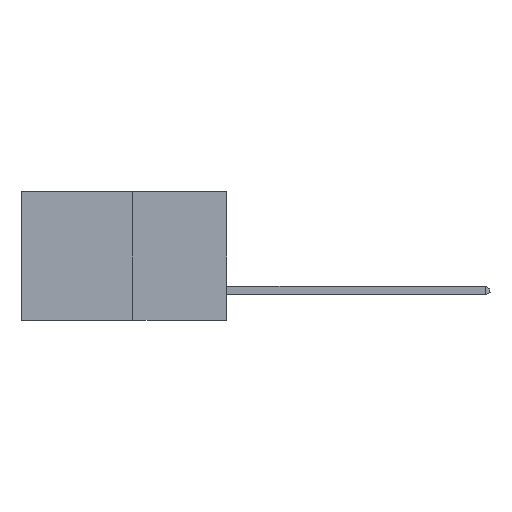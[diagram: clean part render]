
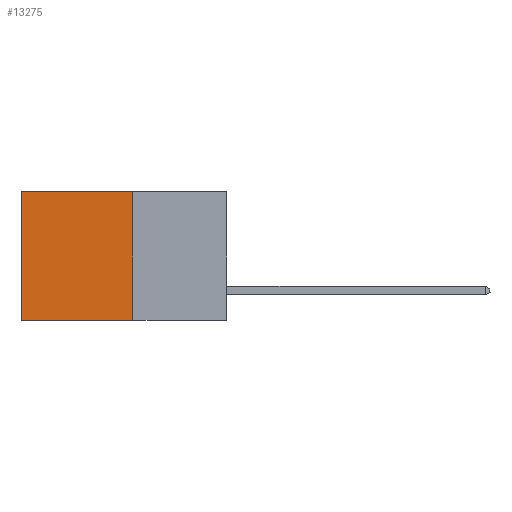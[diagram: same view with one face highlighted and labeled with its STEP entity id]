
A CAD part, left-side view. The second image highlights one B-rep face of the part: STEP entity #13275.
In plain terms, the highlighted planar face has unit normal (-1, 0, 0).
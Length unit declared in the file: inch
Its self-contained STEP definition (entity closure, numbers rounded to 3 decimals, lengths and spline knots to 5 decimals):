
#2609 = ORIENTED_EDGE ( 'NONE', *, *, #19745, .F. ) ;
#3106 = VERTEX_POINT ( 'NONE', #16594 ) ;
#4172 = VECTOR ( 'NONE', #20752, 39.37008 ) ;
#4810 = DIRECTION ( 'NONE',  ( 0., 0., -1. ) ) ;
#5733 = CARTESIAN_POINT ( 'NONE',  ( 0.277, 0.59, 0. ) ) ;
#6549 = CARTESIAN_POINT ( 'NONE',  ( 0.277, 0.27, -0.37 ) ) ;
#6556 = CARTESIAN_POINT ( 'NONE',  ( 0.277, 0.27, 0. ) ) ;
#6880 = ORIENTED_EDGE ( 'NONE', *, *, #17676, .T. ) ;
#8748 = LINE ( 'NONE', #12449, #21718 ) ;
#9411 = LINE ( 'NONE', #9906, #18291 ) ;
#9906 = CARTESIAN_POINT ( 'NONE',  ( 0.277, 0.27, -0.37 ) ) ;
#11186 = VERTEX_POINT ( 'NONE', #5733 ) ;
#11921 = PLANE ( 'NONE',  #19477 ) ;
#12449 = CARTESIAN_POINT ( 'NONE',  ( 0.277, 0.27, -0.37 ) ) ;
#12940 = EDGE_CURVE ( 'NONE', #11186, #3106, #22550, .T. ) ;
#13170 = VECTOR ( 'NONE', #19973, 39.37008 ) ;
#13275 = ADVANCED_FACE ( 'NONE', ( #20073 ), #11921, .F. ) ;
#15099 = DIRECTION ( 'NONE',  ( 0., 1., 0. ) ) ;
#15234 = CARTESIAN_POINT ( 'NONE',  ( 0.277, 0.27, 0. ) ) ;
#15489 = DIRECTION ( 'NONE',  ( 1., 0., 0. ) ) ;
#15617 = ORIENTED_EDGE ( 'NONE', *, *, #16599, .F. ) ;
#16089 = DIRECTION ( 'NONE',  ( 0., 0., -1. ) ) ;
#16594 = CARTESIAN_POINT ( 'NONE',  ( 0.277, 0.59, -0.37 ) ) ;
#16599 = EDGE_CURVE ( 'NONE', #18246, #21351, #8748, .T. ) ;
#17648 = ORIENTED_EDGE ( 'NONE', *, *, #12940, .T. ) ;
#17676 = EDGE_CURVE ( 'NONE', #18246, #11186, #21937, .T. ) ;
#18214 = CARTESIAN_POINT ( 'NONE',  ( 0.277, 0.59, -0.37 ) ) ;
#18246 = VERTEX_POINT ( 'NONE', #15234 ) ;
#18291 = VECTOR ( 'NONE', #15099, 39.37008 ) ;
#19477 = AXIS2_PLACEMENT_3D ( 'NONE', #6549, #15489, #4810 ) ;
#19745 = EDGE_CURVE ( 'NONE', #21351, #3106, #9411, .T. ) ;
#19762 = CARTESIAN_POINT ( 'NONE',  ( 0.277, 0.27, -0.37 ) ) ;
#19973 = DIRECTION ( 'NONE',  ( 0., 0., -1. ) ) ;
#20073 = FACE_OUTER_BOUND ( 'NONE', #20859, .T. ) ;
#20752 = DIRECTION ( 'NONE',  ( 0., 1., 0. ) ) ;
#20859 = EDGE_LOOP ( 'NONE', ( #17648, #2609, #15617, #6880 ) ) ;
#21351 = VERTEX_POINT ( 'NONE', #19762 ) ;
#21718 = VECTOR ( 'NONE', #16089, 39.37008 ) ;
#21937 = LINE ( 'NONE', #6556, #4172 ) ;
#22550 = LINE ( 'NONE', #18214, #13170 ) ;
